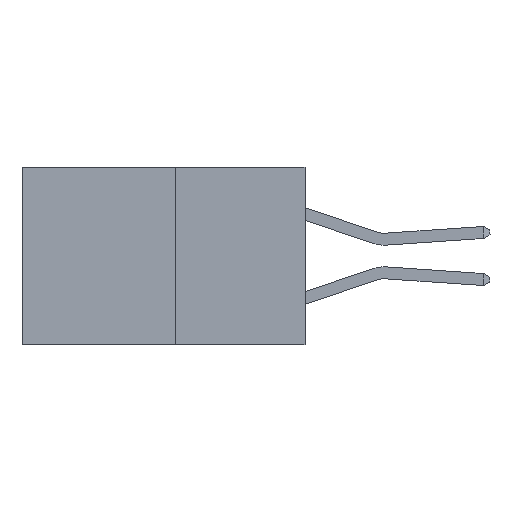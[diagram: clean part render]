
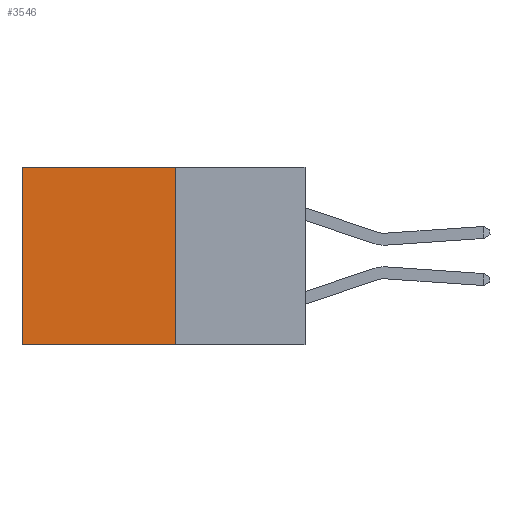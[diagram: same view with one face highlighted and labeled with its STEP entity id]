
A CAD part, left-side view. The second image highlights one B-rep face of the part: STEP entity #3546.
In plain terms, the highlighted planar face has unit normal (-1, 0, 0).
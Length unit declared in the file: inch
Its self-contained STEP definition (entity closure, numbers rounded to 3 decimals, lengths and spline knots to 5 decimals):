
#104 = DIRECTION ( 'NONE',  ( 0., 1., 0. ) ) ;
#360 = VECTOR ( 'NONE', #4066, 39.37008 ) ;
#532 = CARTESIAN_POINT ( 'NONE',  ( 0.277, 0.27, -0.37 ) ) ;
#801 = DIRECTION ( 'NONE',  ( 0., 0., -1. ) ) ;
#849 = CARTESIAN_POINT ( 'NONE',  ( 0.277, 0.59, -0.37 ) ) ;
#1290 = EDGE_LOOP ( 'NONE', ( #9627, #3147, #5458, #8139 ) ) ;
#2746 = LINE ( 'NONE', #4226, #360 ) ;
#2893 = EDGE_CURVE ( 'NONE', #8430, #4396, #3735, .T. ) ;
#2990 = VERTEX_POINT ( 'NONE', #3607 ) ;
#3147 = ORIENTED_EDGE ( 'NONE', *, *, #2893, .F. ) ;
#3546 = ADVANCED_FACE ( 'NONE', ( #11074 ), #5304, .F. ) ;
#3607 = CARTESIAN_POINT ( 'NONE',  ( 0.277, 0.59, 0. ) ) ;
#3735 = LINE ( 'NONE', #5757, #6259 ) ;
#3963 = EDGE_CURVE ( 'NONE', #2990, #4396, #5613, .T. ) ;
#4066 = DIRECTION ( 'NONE',  ( 0., 0., -1. ) ) ;
#4226 = CARTESIAN_POINT ( 'NONE',  ( 0.277, 0.27, -0.37 ) ) ;
#4396 = VERTEX_POINT ( 'NONE', #10716 ) ;
#4558 = CARTESIAN_POINT ( 'NONE',  ( 0.277, 0.27, 0. ) ) ;
#4929 = EDGE_CURVE ( 'NONE', #7024, #8430, #2746, .T. ) ;
#5213 = DIRECTION ( 'NONE',  ( 0., 0., -1. ) ) ;
#5226 = DIRECTION ( 'NONE',  ( 1., 0., 0. ) ) ;
#5278 = CARTESIAN_POINT ( 'NONE',  ( 0.277, 0.27, -0.37 ) ) ;
#5304 = PLANE ( 'NONE',  #9352 ) ;
#5458 = ORIENTED_EDGE ( 'NONE', *, *, #4929, .F. ) ;
#5613 = LINE ( 'NONE', #849, #7536 ) ;
#5689 = DIRECTION ( 'NONE',  ( 0., 1., 0. ) ) ;
#5731 = VECTOR ( 'NONE', #104, 39.37008 ) ;
#5757 = CARTESIAN_POINT ( 'NONE',  ( 0.277, 0.27, -0.37 ) ) ;
#6254 = LINE ( 'NONE', #4558, #5731 ) ;
#6259 = VECTOR ( 'NONE', #5689, 39.37008 ) ;
#7024 = VERTEX_POINT ( 'NONE', #11043 ) ;
#7536 = VECTOR ( 'NONE', #801, 39.37008 ) ;
#8139 = ORIENTED_EDGE ( 'NONE', *, *, #9368, .T. ) ;
#8430 = VERTEX_POINT ( 'NONE', #532 ) ;
#9352 = AXIS2_PLACEMENT_3D ( 'NONE', #5278, #5226, #5213 ) ;
#9368 = EDGE_CURVE ( 'NONE', #7024, #2990, #6254, .T. ) ;
#9627 = ORIENTED_EDGE ( 'NONE', *, *, #3963, .T. ) ;
#10716 = CARTESIAN_POINT ( 'NONE',  ( 0.277, 0.59, -0.37 ) ) ;
#11043 = CARTESIAN_POINT ( 'NONE',  ( 0.277, 0.27, 0. ) ) ;
#11074 = FACE_OUTER_BOUND ( 'NONE', #1290, .T. ) ;
